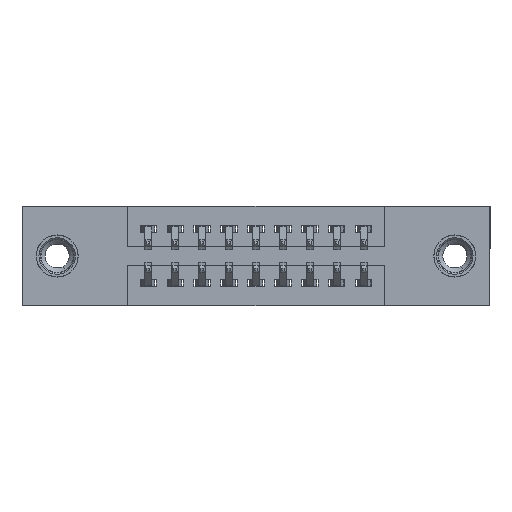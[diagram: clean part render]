
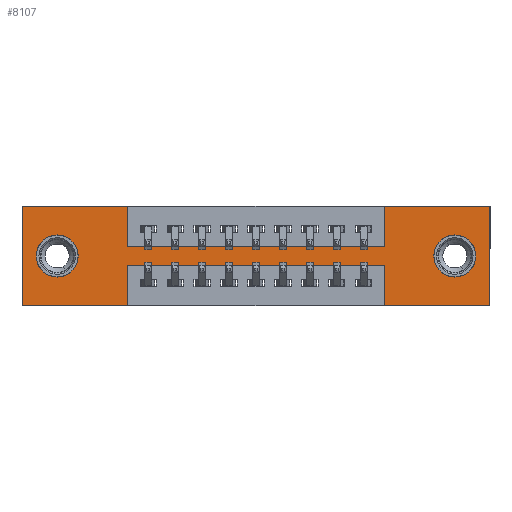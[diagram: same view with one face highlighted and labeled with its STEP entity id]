
A CAD part, front view. The second image highlights one B-rep face of the part: STEP entity #8107.
In plain terms, the highlighted planar face has unit normal (0, -1, 0).
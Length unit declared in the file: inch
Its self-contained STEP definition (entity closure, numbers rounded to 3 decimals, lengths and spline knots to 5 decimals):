
#212 = CARTESIAN_POINT ( 'NONE',  ( 0., 0., 0. ) ) ;
#352 = EDGE_CURVE ( 'NONE', #13334, #7614, #11564, .T. ) ;
#503 = VERTEX_POINT ( 'NONE', #12961 ) ;
#614 = VERTEX_POINT ( 'NONE', #2903 ) ;
#722 = DIRECTION ( 'NONE',  ( 1., 0., 0. ) ) ;
#856 = ORIENTED_EDGE ( 'NONE', *, *, #930, .F. ) ;
#930 = EDGE_CURVE ( 'NONE', #4709, #13508, #14355, .T. ) ;
#1034 = CARTESIAN_POINT ( 'NONE',  ( 1.605, 0., -0.107 ) ) ;
#1181 = EDGE_LOOP ( 'NONE', ( #1933, #2369 ) ) ;
#1246 = EDGE_LOOP ( 'NONE', ( #2806, #6308, #16090, #10060, #16470, #3672, #10450, #13655, #4103, #7495, #856, #7894 ) ) ;
#1530 = CARTESIAN_POINT ( 'NONE',  ( 0., 0., 0. ) ) ;
#1575 = EDGE_CURVE ( 'NONE', #1959, #6737, #4669, .T. ) ;
#1933 = ORIENTED_EDGE ( 'NONE', *, *, #352, .T. ) ;
#1959 = VERTEX_POINT ( 'NONE', #12393 ) ;
#2032 = DIRECTION ( 'NONE',  ( 0., 0., 1. ) ) ;
#2369 = ORIENTED_EDGE ( 'NONE', *, *, #6038, .T. ) ;
#2388 = DIRECTION ( 'NONE',  ( 1., 0., 0. ) ) ;
#2475 = VERTEX_POINT ( 'NONE', #8463 ) ;
#2519 = EDGE_CURVE ( 'NONE', #10338, #2550, #5046, .T. ) ;
#2550 = VERTEX_POINT ( 'NONE', #8147 ) ;
#2675 = LINE ( 'NONE', #8207, #6586 ) ;
#2806 = ORIENTED_EDGE ( 'NONE', *, *, #13034, .F. ) ;
#2903 = CARTESIAN_POINT ( 'NONE',  ( 0.3925, 0., 0. ) ) ;
#2982 = CARTESIAN_POINT ( 'NONE',  ( 1.3425, 0., -0.37 ) ) ;
#3004 = EDGE_CURVE ( 'NONE', #614, #10651, #5029, .T. ) ;
#3068 = FACE_OUTER_BOUND ( 'NONE', #1246, .T. ) ;
#3672 = ORIENTED_EDGE ( 'NONE', *, *, #13585, .F. ) ;
#3690 = CARTESIAN_POINT ( 'NONE',  ( 1.3425, 0., 0. ) ) ;
#3968 = DIRECTION ( 'NONE',  ( -1., 0., 0. ) ) ;
#4103 = ORIENTED_EDGE ( 'NONE', *, *, #3004, .F. ) ;
#4523 = VECTOR ( 'NONE', #8769, 39.37008 ) ;
#4669 = LINE ( 'NONE', #7538, #13427 ) ;
#4709 = VERTEX_POINT ( 'NONE', #5921 ) ;
#4807 = VECTOR ( 'NONE', #8188, 39.37008 ) ;
#5029 = LINE ( 'NONE', #15887, #5454 ) ;
#5046 = CIRCLE ( 'NONE', #14194, 0.078 ) ;
#5282 = VERTEX_POINT ( 'NONE', #7229 ) ;
#5404 = CARTESIAN_POINT ( 'NONE',  ( 0.3925, 0., -0.15 ) ) ;
#5454 = VECTOR ( 'NONE', #8598, 39.37008 ) ;
#5461 = VECTOR ( 'NONE', #15448, 39.37008 ) ;
#5779 = EDGE_CURVE ( 'NONE', #12756, #1959, #12116, .T. ) ;
#5921 = CARTESIAN_POINT ( 'NONE',  ( 0., 0., -0.37 ) ) ;
#6038 = EDGE_CURVE ( 'NONE', #7614, #13334, #15062, .T. ) ;
#6158 = VECTOR ( 'NONE', #9366, 39.37008 ) ;
#6283 = DIRECTION ( 'NONE',  ( -1., 0., 0. ) ) ;
#6308 = ORIENTED_EDGE ( 'NONE', *, *, #1575, .F. ) ;
#6385 = CARTESIAN_POINT ( 'NONE',  ( 1.3425, 0., -0.37 ) ) ;
#6501 = CARTESIAN_POINT ( 'NONE',  ( 1.735, 0., -0.37 ) ) ;
#6547 = CARTESIAN_POINT ( 'NONE',  ( 0.13, 0., -0.185 ) ) ;
#6586 = VECTOR ( 'NONE', #9581, 39.37008 ) ;
#6737 = VERTEX_POINT ( 'NONE', #10895 ) ;
#6802 = DIRECTION ( 'NONE',  ( 0., 1., 0. ) ) ;
#6954 = FACE_BOUND ( 'NONE', #8070, .T. ) ;
#7204 = VECTOR ( 'NONE', #2388, 39.37008 ) ;
#7229 = CARTESIAN_POINT ( 'NONE',  ( 1.735, 0., 0. ) ) ;
#7240 = DIRECTION ( 'NONE',  ( 0., 0., -1. ) ) ;
#7419 = VECTOR ( 'NONE', #722, 39.37008 ) ;
#7495 = ORIENTED_EDGE ( 'NONE', *, *, #12066, .F. ) ;
#7538 = CARTESIAN_POINT ( 'NONE',  ( 0.3925, 0., -0.22 ) ) ;
#7614 = VERTEX_POINT ( 'NONE', #8787 ) ;
#7806 = DIRECTION ( 'NONE',  ( 0., 0., 1. ) ) ;
#7894 = ORIENTED_EDGE ( 'NONE', *, *, #15611, .F. ) ;
#8070 = EDGE_LOOP ( 'NONE', ( #12553, #15722 ) ) ;
#8098 = CARTESIAN_POINT ( 'NONE',  ( 1.735, 0., 0. ) ) ;
#8100 = AXIS2_PLACEMENT_3D ( 'NONE', #14743, #15946, #8653 ) ;
#8104 = CARTESIAN_POINT ( 'NONE',  ( 0., 0., -0.37 ) ) ;
#8107 = ADVANCED_FACE ( 'NONE', ( #9900, #6954, #3068 ), #11124, .T. ) ;
#8147 = CARTESIAN_POINT ( 'NONE',  ( 0.13, 0., -0.107 ) ) ;
#8166 = VECTOR ( 'NONE', #15412, 39.37008 ) ;
#8188 = DIRECTION ( 'NONE',  ( 1., 0., 0. ) ) ;
#8207 = CARTESIAN_POINT ( 'NONE',  ( 0.3925, 0., -0.37 ) ) ;
#8294 = LINE ( 'NONE', #16050, #4523 ) ;
#8463 = CARTESIAN_POINT ( 'NONE',  ( 1.3425, 0., -0.15 ) ) ;
#8592 = AXIS2_PLACEMENT_3D ( 'NONE', #14177, #6802, #15377 ) ;
#8598 = DIRECTION ( 'NONE',  ( 0., 0., -1. ) ) ;
#8653 = DIRECTION ( 'NONE',  ( 0., 0., -1. ) ) ;
#8769 = DIRECTION ( 'NONE',  ( 0., 0., 1. ) ) ;
#8787 = CARTESIAN_POINT ( 'NONE',  ( 1.605, 0., -0.263 ) ) ;
#8804 = EDGE_CURVE ( 'NONE', #5282, #15585, #15943, .T. ) ;
#9366 = DIRECTION ( 'NONE',  ( 0., 0., -1. ) ) ;
#9388 = CARTESIAN_POINT ( 'NONE',  ( 0.13, 0., -0.185 ) ) ;
#9581 = DIRECTION ( 'NONE',  ( 0., 0., -1. ) ) ;
#9808 = CARTESIAN_POINT ( 'NONE',  ( 0.13, 0., -0.263 ) ) ;
#9868 = EDGE_CURVE ( 'NONE', #2475, #15002, #8294, .T. ) ;
#9900 = FACE_BOUND ( 'NONE', #1181, .T. ) ;
#10060 = ORIENTED_EDGE ( 'NONE', *, *, #14005, .F. ) ;
#10135 = CARTESIAN_POINT ( 'NONE',  ( 0.3925, 0., -0.15 ) ) ;
#10338 = VERTEX_POINT ( 'NONE', #9808 ) ;
#10450 = ORIENTED_EDGE ( 'NONE', *, *, #9868, .F. ) ;
#10599 = EDGE_CURVE ( 'NONE', #2550, #10338, #14746, .T. ) ;
#10651 = VERTEX_POINT ( 'NONE', #5404 ) ;
#10895 = CARTESIAN_POINT ( 'NONE',  ( 0.3925, 0., -0.22 ) ) ;
#11124 = PLANE ( 'NONE',  #8100 ) ;
#11154 = AXIS2_PLACEMENT_3D ( 'NONE', #12595, #14265, #7240 ) ;
#11163 = VECTOR ( 'NONE', #2032, 39.37008 ) ;
#11564 = CIRCLE ( 'NONE', #11154, 0.078 ) ;
#12066 = EDGE_CURVE ( 'NONE', #13508, #614, #13947, .T. ) ;
#12116 = LINE ( 'NONE', #2982, #5461 ) ;
#12393 = CARTESIAN_POINT ( 'NONE',  ( 1.3425, 0., -0.22 ) ) ;
#12553 = ORIENTED_EDGE ( 'NONE', *, *, #10599, .T. ) ;
#12595 = CARTESIAN_POINT ( 'NONE',  ( 1.605, 0., -0.185 ) ) ;
#12731 = EDGE_CURVE ( 'NONE', #10651, #2475, #13371, .T. ) ;
#12747 = CARTESIAN_POINT ( 'NONE',  ( 0., 0., -0.37 ) ) ;
#12748 = VECTOR ( 'NONE', #3968, 39.37008 ) ;
#12756 = VERTEX_POINT ( 'NONE', #6385 ) ;
#12961 = CARTESIAN_POINT ( 'NONE',  ( 0.3925, 0., -0.37 ) ) ;
#13034 = EDGE_CURVE ( 'NONE', #6737, #503, #2675, .T. ) ;
#13334 = VERTEX_POINT ( 'NONE', #1034 ) ;
#13371 = LINE ( 'NONE', #10135, #7204 ) ;
#13427 = VECTOR ( 'NONE', #6283, 39.37008 ) ;
#13508 = VERTEX_POINT ( 'NONE', #15324 ) ;
#13585 = EDGE_CURVE ( 'NONE', #15002, #5282, #14306, .T. ) ;
#13655 = ORIENTED_EDGE ( 'NONE', *, *, #12731, .F. ) ;
#13947 = LINE ( 'NONE', #15894, #7419 ) ;
#14005 = EDGE_CURVE ( 'NONE', #15585, #12756, #15028, .T. ) ;
#14177 = CARTESIAN_POINT ( 'NONE',  ( 1.605, 0., -0.185 ) ) ;
#14194 = AXIS2_PLACEMENT_3D ( 'NONE', #9388, #14538, #15918 ) ;
#14265 = DIRECTION ( 'NONE',  ( 0., 1., 0. ) ) ;
#14306 = LINE ( 'NONE', #212, #4807 ) ;
#14355 = LINE ( 'NONE', #1530, #11163 ) ;
#14538 = DIRECTION ( 'NONE',  ( 0., 1., 0. ) ) ;
#14649 = AXIS2_PLACEMENT_3D ( 'NONE', #6547, #15130, #7806 ) ;
#14743 = CARTESIAN_POINT ( 'NONE',  ( 0., 0., -0.37 ) ) ;
#14746 = CIRCLE ( 'NONE', #14649, 0.078 ) ;
#15002 = VERTEX_POINT ( 'NONE', #3690 ) ;
#15028 = LINE ( 'NONE', #8104, #8166 ) ;
#15062 = CIRCLE ( 'NONE', #8592, 0.078 ) ;
#15130 = DIRECTION ( 'NONE',  ( 0., 1., 0. ) ) ;
#15324 = CARTESIAN_POINT ( 'NONE',  ( 0., 0., 0. ) ) ;
#15377 = DIRECTION ( 'NONE',  ( 0., 0., -1. ) ) ;
#15412 = DIRECTION ( 'NONE',  ( -1., 0., 0. ) ) ;
#15448 = DIRECTION ( 'NONE',  ( 0., 0., 1. ) ) ;
#15547 = LINE ( 'NONE', #12747, #12748 ) ;
#15585 = VERTEX_POINT ( 'NONE', #6501 ) ;
#15611 = EDGE_CURVE ( 'NONE', #503, #4709, #15547, .T. ) ;
#15722 = ORIENTED_EDGE ( 'NONE', *, *, #2519, .T. ) ;
#15887 = CARTESIAN_POINT ( 'NONE',  ( 0.3925, 0., 0. ) ) ;
#15894 = CARTESIAN_POINT ( 'NONE',  ( 0., 0., 0. ) ) ;
#15918 = DIRECTION ( 'NONE',  ( 0., 0., 1. ) ) ;
#15943 = LINE ( 'NONE', #8098, #6158 ) ;
#15946 = DIRECTION ( 'NONE',  ( 0., -1., 0. ) ) ;
#16050 = CARTESIAN_POINT ( 'NONE',  ( 1.3425, 0., 0. ) ) ;
#16090 = ORIENTED_EDGE ( 'NONE', *, *, #5779, .F. ) ;
#16470 = ORIENTED_EDGE ( 'NONE', *, *, #8804, .F. ) ;
